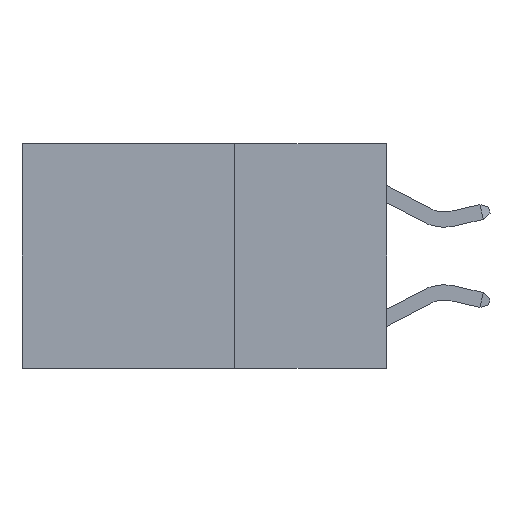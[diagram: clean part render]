
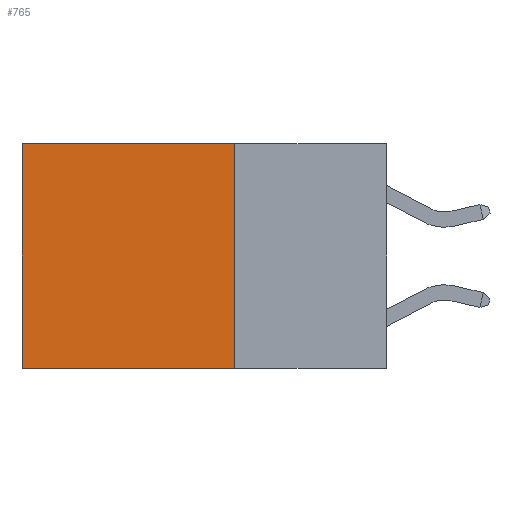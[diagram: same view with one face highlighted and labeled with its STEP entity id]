
A CAD part, left-side view. The second image highlights one B-rep face of the part: STEP entity #765.
In plain terms, the highlighted planar face has unit normal (-1, 0, 0).
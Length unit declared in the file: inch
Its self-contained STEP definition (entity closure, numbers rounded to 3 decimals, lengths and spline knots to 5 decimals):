
#555 = ORIENTED_EDGE ( 'NONE', *, *, #9337, .F. ) ;
#765 = ADVANCED_FACE ( 'NONE', ( #3509 ), #7882, .F. ) ;
#786 = EDGE_CURVE ( 'NONE', #4786, #8332, #5013, .T. ) ;
#954 = LINE ( 'NONE', #6971, #4867 ) ;
#1218 = AXIS2_PLACEMENT_3D ( 'NONE', #8786, #2045, #2091 ) ;
#1335 = ORIENTED_EDGE ( 'NONE', *, *, #1599, .F. ) ;
#1508 = DIRECTION ( 'NONE',  ( 0., 1., 0. ) ) ;
#1552 = DIRECTION ( 'NONE',  ( 0., 0., -1. ) ) ;
#1599 = EDGE_CURVE ( 'NONE', #6527, #8332, #4447, .T. ) ;
#1866 = VECTOR ( 'NONE', #1508, 39.37008 ) ;
#2045 = DIRECTION ( 'NONE',  ( 1., 0., 0. ) ) ;
#2091 = DIRECTION ( 'NONE',  ( 0., 0., -1. ) ) ;
#2285 = LINE ( 'NONE', #5295, #4648 ) ;
#2356 = VERTEX_POINT ( 'NONE', #9637 ) ;
#2820 = DIRECTION ( 'NONE',  ( 0., 0., -1. ) ) ;
#2869 = CARTESIAN_POINT ( 'NONE',  ( 0.2625, 0.25, -0.37 ) ) ;
#3374 = EDGE_CURVE ( 'NONE', #2356, #4786, #954, .T. ) ;
#3509 = FACE_OUTER_BOUND ( 'NONE', #4963, .T. ) ;
#3746 = VECTOR ( 'NONE', #2820, 39.37008 ) ;
#3846 = CARTESIAN_POINT ( 'NONE',  ( 0.2625, 0.25, -0.37 ) ) ;
#3882 = CARTESIAN_POINT ( 'NONE',  ( 0.2625, 0.6, -0.37 ) ) ;
#4447 = LINE ( 'NONE', #2869, #1866 ) ;
#4648 = VECTOR ( 'NONE', #1552, 39.37008 ) ;
#4786 = VERTEX_POINT ( 'NONE', #6484 ) ;
#4867 = VECTOR ( 'NONE', #9235, 39.37008 ) ;
#4963 = EDGE_LOOP ( 'NONE', ( #9607, #1335, #555, #6978 ) ) ;
#5013 = LINE ( 'NONE', #8630, #3746 ) ;
#5295 = CARTESIAN_POINT ( 'NONE',  ( 0.2625, 0.25, 0. ) ) ;
#6484 = CARTESIAN_POINT ( 'NONE',  ( 0.2625, 0.6, 0. ) ) ;
#6527 = VERTEX_POINT ( 'NONE', #3846 ) ;
#6971 = CARTESIAN_POINT ( 'NONE',  ( 0.2625, 0.25, 0. ) ) ;
#6978 = ORIENTED_EDGE ( 'NONE', *, *, #3374, .T. ) ;
#7882 = PLANE ( 'NONE',  #1218 ) ;
#8332 = VERTEX_POINT ( 'NONE', #3882 ) ;
#8630 = CARTESIAN_POINT ( 'NONE',  ( 0.2625, 0.6, 0. ) ) ;
#8786 = CARTESIAN_POINT ( 'NONE',  ( 0.2625, 0.25, 0. ) ) ;
#9235 = DIRECTION ( 'NONE',  ( 0., 1., 0. ) ) ;
#9337 = EDGE_CURVE ( 'NONE', #2356, #6527, #2285, .T. ) ;
#9607 = ORIENTED_EDGE ( 'NONE', *, *, #786, .T. ) ;
#9637 = CARTESIAN_POINT ( 'NONE',  ( 0.2625, 0.25, 0. ) ) ;
